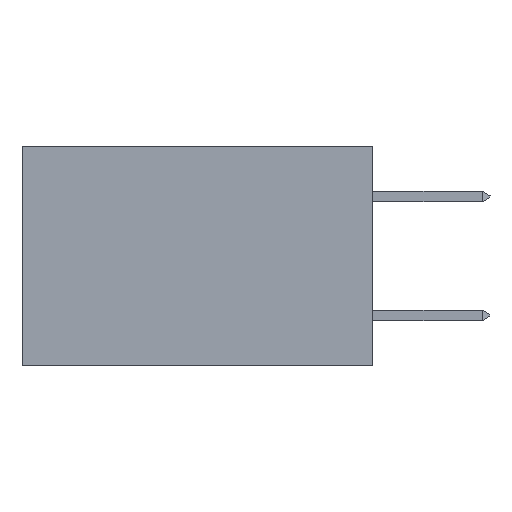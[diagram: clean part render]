
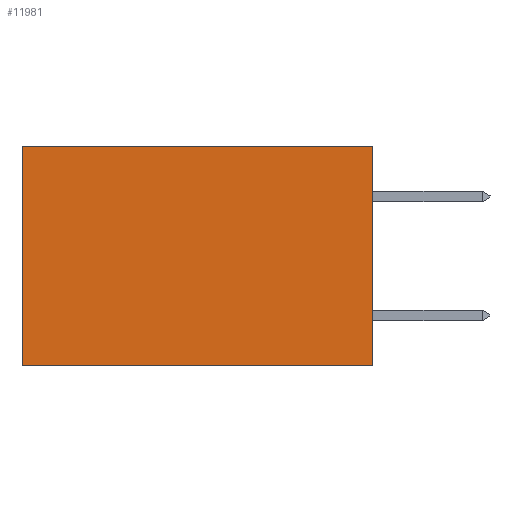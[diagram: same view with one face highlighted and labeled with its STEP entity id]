
A CAD part, left-side view. The second image highlights one B-rep face of the part: STEP entity #11981.
In plain terms, the highlighted planar face has unit normal (-1, 0, 0).
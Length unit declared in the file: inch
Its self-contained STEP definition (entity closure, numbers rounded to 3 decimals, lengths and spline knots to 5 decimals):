
#3707 = VERTEX_POINT ( 'NONE', #11435 ) ;
#3823 = CARTESIAN_POINT ( 'NONE',  ( 0.277, 0.59, -0.37 ) ) ;
#4191 = EDGE_CURVE ( 'NONE', #3707, #22895, #9473, .T. ) ;
#4315 = VECTOR ( 'NONE', #24236, 39.37008 ) ;
#4480 = EDGE_LOOP ( 'NONE', ( #8128, #8425, #8567, #8931 ) ) ;
#4904 = FACE_OUTER_BOUND ( 'NONE', #4480, .T. ) ;
#5663 = EDGE_CURVE ( 'NONE', #20880, #3707, #23246, .T. ) ;
#7098 = VECTOR ( 'NONE', #19212, 39.37008 ) ;
#7905 = CARTESIAN_POINT ( 'NONE',  ( 0.277, 0.59, -0.37 ) ) ;
#8128 = ORIENTED_EDGE ( 'NONE', *, *, #19536, .T. ) ;
#8195 = VECTOR ( 'NONE', #11850, 39.37008 ) ;
#8336 = PLANE ( 'NONE',  #16735 ) ;
#8417 = DIRECTION ( 'NONE',  ( 1., 0., 0. ) ) ;
#8425 = ORIENTED_EDGE ( 'NONE', *, *, #4191, .F. ) ;
#8567 = ORIENTED_EDGE ( 'NONE', *, *, #5663, .F. ) ;
#8931 = ORIENTED_EDGE ( 'NONE', *, *, #19555, .T. ) ;
#9473 = LINE ( 'NONE', #24183, #4315 ) ;
#9667 = CARTESIAN_POINT ( 'NONE',  ( 0.277, 0.59, 0. ) ) ;
#9771 = DIRECTION ( 'NONE',  ( 0., 1., 0. ) ) ;
#11435 = CARTESIAN_POINT ( 'NONE',  ( 0.277, 0., -0.37 ) ) ;
#11850 = DIRECTION ( 'NONE',  ( 0., 0., -1. ) ) ;
#11981 = ADVANCED_FACE ( 'NONE', ( #4904 ), #8336, .F. ) ;
#12240 = LINE ( 'NONE', #3823, #7098 ) ;
#12459 = CARTESIAN_POINT ( 'NONE',  ( 0.277, 0., -0.37 ) ) ;
#12855 = VECTOR ( 'NONE', #9771, 39.37008 ) ;
#16735 = AXIS2_PLACEMENT_3D ( 'NONE', #19837, #8417, #21666 ) ;
#16769 = LINE ( 'NONE', #21139, #12855 ) ;
#17266 = VERTEX_POINT ( 'NONE', #9667 ) ;
#19212 = DIRECTION ( 'NONE',  ( 0., 0., -1. ) ) ;
#19536 = EDGE_CURVE ( 'NONE', #17266, #22895, #12240, .T. ) ;
#19555 = EDGE_CURVE ( 'NONE', #20880, #17266, #16769, .T. ) ;
#19837 = CARTESIAN_POINT ( 'NONE',  ( 0.277, 0., -0.37 ) ) ;
#20880 = VERTEX_POINT ( 'NONE', #22827 ) ;
#21139 = CARTESIAN_POINT ( 'NONE',  ( 0.277, 0., 0. ) ) ;
#21666 = DIRECTION ( 'NONE',  ( 0., 0., -1. ) ) ;
#22827 = CARTESIAN_POINT ( 'NONE',  ( 0.277, 0., 0. ) ) ;
#22895 = VERTEX_POINT ( 'NONE', #7905 ) ;
#23246 = LINE ( 'NONE', #12459, #8195 ) ;
#24183 = CARTESIAN_POINT ( 'NONE',  ( 0.277, 0., -0.37 ) ) ;
#24236 = DIRECTION ( 'NONE',  ( 0., 1., 0. ) ) ;
